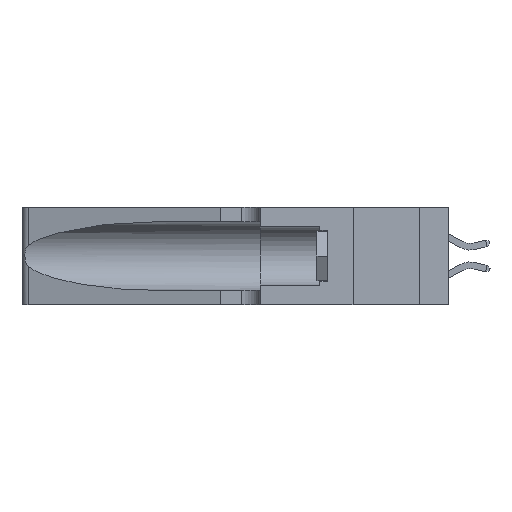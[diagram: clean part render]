
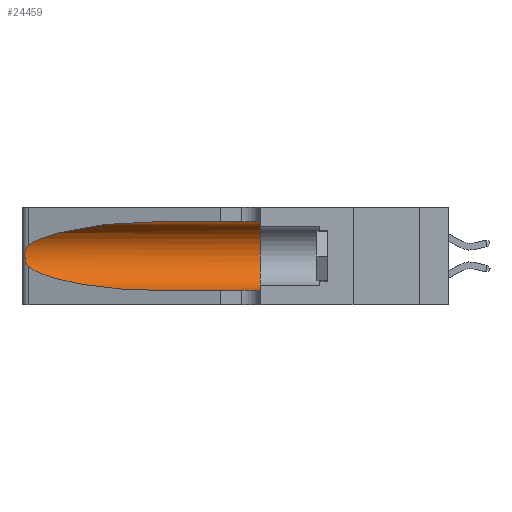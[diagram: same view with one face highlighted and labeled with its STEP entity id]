
A CAD part, left-side view. The second image highlights one B-rep face of the part: STEP entity #24459.
In plain terms, the highlighted cylindrical face has radius 3.308 mm (diameter 6.617 mm), a partial arc.
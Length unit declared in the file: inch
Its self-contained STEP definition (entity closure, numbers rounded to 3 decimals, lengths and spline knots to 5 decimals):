
#105 = DIRECTION ( 'NONE',  ( 0., 0., -1. ) ) ;
#373 = CARTESIAN_POINT ( 'NONE',  ( 0.25555, 1.22994, 0.2215 ) ) ;
#733 = AXIS2_PLACEMENT_3D ( 'NONE', #16106, #20060, #6189 ) ;
#2160 = CARTESIAN_POINT ( 'NONE',  ( 0.18966, 0.96281, 0.31525 ) ) ;
#2460 = DIRECTION ( 'NONE',  ( 0., -1., 0. ) ) ;
#2499 = B_SPLINE_CURVE_WITH_KNOTS ( 'NONE', 3,
 ( #7564, #373, #11289, #15938, #8053, #13940, #6226, #5894, #23876, #4059, #21989, #8133, #25700, #7031 ),
 .UNSPECIFIED., .F., .F.,
 ( 4, 2, 2, 2, 2, 2, 4 ),
 ( 0., 0.00027, 0.00053, 0.00107, 0.0016, 0.00187, 0.00214 ),
 .UNSPECIFIED. ) ;
#2585 = CARTESIAN_POINT ( 'NONE',  ( 0.18966, 0.96281, 0.05475 ) ) ;
#2677 = VERTEX_POINT ( 'NONE', #4629 ) ;
#2781 = ORIENTED_EDGE ( 'NONE', *, *, #5616, .T. ) ;
#3029 = EDGE_CURVE ( 'NONE', #7580, #22605, #20210, .T. ) ;
#3246 = CARTESIAN_POINT ( 'NONE',  ( 0.1305, 0.72297, 0.31525 ) ) ;
#3679 = EDGE_CURVE ( 'NONE', #22605, #10194, #5838, .T. ) ;
#4059 = CARTESIAN_POINT ( 'NONE',  ( 0.25856, 1.23593, 0.16098 ) ) ;
#4134 = CARTESIAN_POINT ( 'NONE',  ( 0.25487, 1.22718, 0.22369 ) ) ;
#4629 = CARTESIAN_POINT ( 'NONE',  ( 0.1305, 0.72297, 0.05475 ) ) ;
#5392 = EDGE_CURVE ( 'NONE', #7580, #5726, #15651, .T. ) ;
#5616 = EDGE_CURVE ( 'NONE', #2677, #10194, #11367, .T. ) ;
#5726 = VERTEX_POINT ( 'NONE', #18289 ) ;
#5838 = CIRCLE ( 'NONE', #733, 0.13025 ) ;
#5894 = CARTESIAN_POINT ( 'NONE',  ( 0.26075, 1.23896, 0.178 ) ) ;
#6189 = DIRECTION ( 'NONE',  ( 0., 0., 1. ) ) ;
#6226 = CARTESIAN_POINT ( 'NONE',  ( 0.26075, 1.23896, 0.19203 ) ) ;
#6440 = CARTESIAN_POINT ( 'NONE',  ( 0.25487, 1.22718, 0.14631 ) ) ;
#6583 = CARTESIAN_POINT ( 'NONE',  ( 0.25487, 1.22718, 0.14631 ) ) ;
#7031 = CARTESIAN_POINT ( 'NONE',  ( 0.25487, 1.22718, 0.14631 ) ) ;
#7564 = CARTESIAN_POINT ( 'NONE',  ( 0.25487, 1.22718, 0.22369 ) ) ;
#7580 = VERTEX_POINT ( 'NONE', #3246 ) ;
#8053 = CARTESIAN_POINT ( 'NONE',  ( 0.25854, 1.2359, 0.20912 ) ) ;
#8118 = CYLINDRICAL_SURFACE ( 'NONE', #13600, 0.13025 ) ;
#8133 = CARTESIAN_POINT ( 'NONE',  ( 0.25639, 1.23186, 0.15144 ) ) ;
#8321 = CARTESIAN_POINT ( 'NONE',  ( 0.1305, 0.72297, 0.05475 ) ) ;
#10194 = VERTEX_POINT ( 'NONE', #22488 ) ;
#10586 = DIRECTION ( 'NONE',  ( 0., -1., 0. ) ) ;
#11116 = ORIENTED_EDGE ( 'NONE', *, *, #17429, .T. ) ;
#11289 = CARTESIAN_POINT ( 'NONE',  ( 0.25639, 1.23184, 0.21858 ) ) ;
#11367 = LINE ( 'NONE', #18085, #18213 ) ;
#12050 = ORIENTED_EDGE ( 'NONE', *, *, #25662, .T. ) ;
#12481 = VECTOR ( 'NONE', #10586, 39.37008 ) ;
#12802 = ORIENTED_EDGE ( 'NONE', *, *, #3679, .F. ) ;
#13600 = AXIS2_PLACEMENT_3D ( 'NONE', #16183, #2460, #105 ) ;
#13940 = CARTESIAN_POINT ( 'NONE',  ( 0.26018, 1.23835, 0.19895 ) ) ;
#14443 = CARTESIAN_POINT ( 'NONE',  ( 0.1305, 1.61858, 0.31525 ) ) ;
#14648 =( BOUNDED_CURVE ( )  B_SPLINE_CURVE ( 3, ( #6583, #22239, #2585, #8321 ),
 .UNSPECIFIED., .F., .T. ) 
 B_SPLINE_CURVE_WITH_KNOTS ( ( 4, 4 ),
 ( 3.44316, 4.71239 ),
 .UNSPECIFIED. ) 
 CURVE ( )  GEOMETRIC_REPRESENTATION_ITEM ( )  RATIONAL_B_SPLINE_CURVE ( ( 1., 0.87, 0.87, 1. ) ) 
 REPRESENTATION_ITEM ( '' )  );
#15021 = VERTEX_POINT ( 'NONE', #6440 ) ;
#15651 =( BOUNDED_CURVE ( )  B_SPLINE_CURVE ( 3, ( #20169, #2160, #16131, #4134 ),
 .UNSPECIFIED., .F., .F. ) 
 B_SPLINE_CURVE_WITH_KNOTS ( ( 4, 4 ),
 ( 1.5708, 2.84003 ),
 .UNSPECIFIED. ) 
 CURVE ( )  GEOMETRIC_REPRESENTATION_ITEM ( )  RATIONAL_B_SPLINE_CURVE ( ( 1., 0.87, 0.87, 1. ) ) 
 REPRESENTATION_ITEM ( '' )  );
#15918 = EDGE_LOOP ( 'NONE', ( #15990, #11116, #12050, #2781, #12802, #25328 ) ) ;
#15938 = CARTESIAN_POINT ( 'NONE',  ( 0.25787, 1.23484, 0.2124 ) ) ;
#15990 = ORIENTED_EDGE ( 'NONE', *, *, #5392, .T. ) ;
#16106 = CARTESIAN_POINT ( 'NONE',  ( 0.1305, 0.35, 0.185 ) ) ;
#16131 = CARTESIAN_POINT ( 'NONE',  ( 0.2373, 1.15595, 0.28018 ) ) ;
#16183 = CARTESIAN_POINT ( 'NONE',  ( 0.1305, 1.61858, 0.185 ) ) ;
#16367 = DIRECTION ( 'NONE',  ( 0., -1., 0. ) ) ;
#17429 = EDGE_CURVE ( 'NONE', #5726, #15021, #2499, .T. ) ;
#18085 = CARTESIAN_POINT ( 'NONE',  ( 0.1305, 1.61858, 0.05475 ) ) ;
#18213 = VECTOR ( 'NONE', #16367, 39.37008 ) ;
#18289 = CARTESIAN_POINT ( 'NONE',  ( 0.25487, 1.22718, 0.22369 ) ) ;
#20060 = DIRECTION ( 'NONE',  ( 0., 1., 0. ) ) ;
#20169 = CARTESIAN_POINT ( 'NONE',  ( 0.1305, 0.72297, 0.31525 ) ) ;
#20210 = LINE ( 'NONE', #14443, #12481 ) ;
#20914 = FACE_OUTER_BOUND ( 'NONE', #15918, .T. ) ;
#21989 = CARTESIAN_POINT ( 'NONE',  ( 0.25789, 1.23486, 0.15765 ) ) ;
#22239 = CARTESIAN_POINT ( 'NONE',  ( 0.2373, 1.15595, 0.08982 ) ) ;
#22488 = CARTESIAN_POINT ( 'NONE',  ( 0.1305, 0.35, 0.05475 ) ) ;
#22605 = VERTEX_POINT ( 'NONE', #22620 ) ;
#22620 = CARTESIAN_POINT ( 'NONE',  ( 0.1305, 0.35, 0.31525 ) ) ;
#23876 = CARTESIAN_POINT ( 'NONE',  ( 0.26017, 1.23833, 0.17102 ) ) ;
#24459 = ADVANCED_FACE ( 'NONE', ( #20914 ), #8118, .F. ) ;
#25328 = ORIENTED_EDGE ( 'NONE', *, *, #3029, .F. ) ;
#25662 = EDGE_CURVE ( 'NONE', #15021, #2677, #14648, .T. ) ;
#25700 = CARTESIAN_POINT ( 'NONE',  ( 0.25555, 1.22993, 0.14849 ) ) ;
